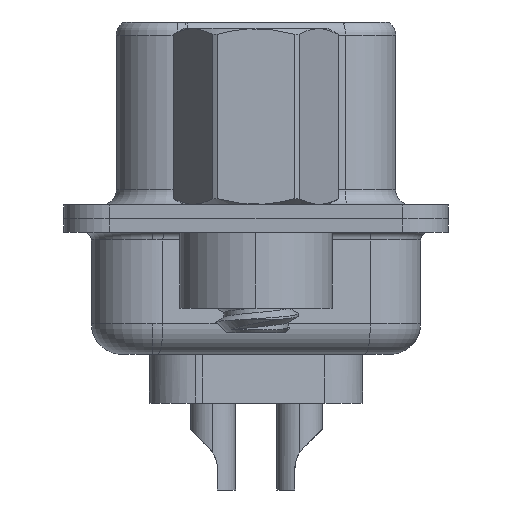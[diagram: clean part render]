
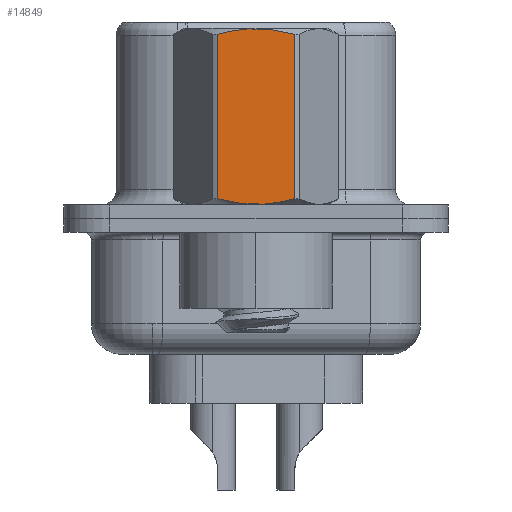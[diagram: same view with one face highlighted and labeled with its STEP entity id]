
A CAD part, left-side view. The second image highlights one B-rep face of the part: STEP entity #14849.
In plain terms, the highlighted planar face has unit normal (-1, 0, 0).
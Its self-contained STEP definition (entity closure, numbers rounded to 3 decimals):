
#554 = VECTOR ( 'NONE', #30911, 1000. ) ;
#1548 = ORIENTED_EDGE ( 'NONE', *, *, #30494, .T. ) ;
#2307 = DIRECTION ( 'NONE',  ( 0., -1., 0. ) ) ;
#3240 = VERTEX_POINT ( 'NONE', #31579 ) ;
#3548 = B_SPLINE_CURVE_WITH_KNOTS ( 'NONE', 3,
 ( #26288, #14529, #26446, #4551, #21928, #31749, #11772, #9682, #9529, #16793 ),
 .UNSPECIFIED., .F., .F.,
 ( 4, 2, 2, 2, 4 ),
 ( 0.001, 0.002, 0.002, 0.003, 0.004 ),
 .UNSPECIFIED. ) ;
#3938 = B_SPLINE_CURVE_WITH_KNOTS ( 'NONE', 3,
 ( #23975, #7053, #26225, #16888, #11562, #16259, #19156, #4168, #31684, #28947 ),
 .UNSPECIFIED., .F., .F.,
 ( 4, 2, 2, 2, 4 ),
 ( 0.003, 0.003, 0.004, 0.004, 0.005 ),
 .UNSPECIFIED. ) ;
#4168 = CARTESIAN_POINT ( 'NONE',  ( -2.381, -0.858, 0.55 ) ) ;
#4551 = CARTESIAN_POINT ( 'NONE',  ( -2.381, -0.432, 6.215 ) ) ;
#5986 = CARTESIAN_POINT ( 'NONE',  ( -2.381, 1.273, 3.792 ) ) ;
#6294 = ORIENTED_EDGE ( 'NONE', *, *, #14105, .T. ) ;
#7053 = CARTESIAN_POINT ( 'NONE',  ( -2.381, 1.065, 0.596 ) ) ;
#7662 = EDGE_LOOP ( 'NONE', ( #6294, #1548, #12717, #27139 ) ) ;
#9517 = PLANE ( 'NONE',  #10542 ) ;
#9529 = CARTESIAN_POINT ( 'NONE',  ( -2.381, 1.065, 6.104 ) ) ;
#9682 = CARTESIAN_POINT ( 'NONE',  ( -2.381, 0.853, 6.151 ) ) ;
#10542 = AXIS2_PLACEMENT_3D ( 'NONE', #26901, #29155, #2307 ) ;
#11562 = CARTESIAN_POINT ( 'NONE',  ( -2.381, 0.215, 0.468 ) ) ;
#11772 = CARTESIAN_POINT ( 'NONE',  ( -2.381, 0.428, 6.215 ) ) ;
#12717 = ORIENTED_EDGE ( 'NONE', *, *, #28779, .T. ) ;
#14105 = EDGE_CURVE ( 'NONE', #3240, #20142, #3938, .T. ) ;
#14252 = CARTESIAN_POINT ( 'NONE',  ( -2.381, -1.273, 6.048 ) ) ;
#14529 = CARTESIAN_POINT ( 'NONE',  ( -2.381, -1.066, 6.104 ) ) ;
#14849 = ADVANCED_FACE ( 'NONE', ( #19507 ), #9517, .T. ) ;
#15960 = LINE ( 'NONE', #5986, #554 ) ;
#15962 = CARTESIAN_POINT ( 'NONE',  ( -2.381, 1.273, 6.048 ) ) ;
#16259 = CARTESIAN_POINT ( 'NONE',  ( -2.381, -0.215, 0.468 ) ) ;
#16793 = CARTESIAN_POINT ( 'NONE',  ( -2.381, 1.273, 6.048 ) ) ;
#16868 = VERTEX_POINT ( 'NONE', #15962 ) ;
#16888 = CARTESIAN_POINT ( 'NONE',  ( -2.381, 0.428, 0.485 ) ) ;
#17293 = LINE ( 'NONE', #27558, #22139 ) ;
#18986 = CARTESIAN_POINT ( 'NONE',  ( -2.381, -1.273, 0.652 ) ) ;
#19156 = CARTESIAN_POINT ( 'NONE',  ( -2.381, -0.432, 0.485 ) ) ;
#19507 = FACE_OUTER_BOUND ( 'NONE', #7662, .T. ) ;
#20142 = VERTEX_POINT ( 'NONE', #18986 ) ;
#21928 = CARTESIAN_POINT ( 'NONE',  ( -2.381, -0.215, 6.232 ) ) ;
#22139 = VECTOR ( 'NONE', #27083, 1000. ) ;
#23975 = CARTESIAN_POINT ( 'NONE',  ( -2.381, 1.273, 0.652 ) ) ;
#25932 = VERTEX_POINT ( 'NONE', #14252 ) ;
#26225 = CARTESIAN_POINT ( 'NONE',  ( -2.381, 0.853, 0.549 ) ) ;
#26288 = CARTESIAN_POINT ( 'NONE',  ( -2.381, -1.273, 6.048 ) ) ;
#26446 = CARTESIAN_POINT ( 'NONE',  ( -2.381, -0.858, 6.15 ) ) ;
#26901 = CARTESIAN_POINT ( 'NONE',  ( -2.381, 1.375, -3.75 ) ) ;
#27083 = DIRECTION ( 'NONE',  ( 0., 0., 1. ) ) ;
#27139 = ORIENTED_EDGE ( 'NONE', *, *, #29092, .T. ) ;
#27558 = CARTESIAN_POINT ( 'NONE',  ( -2.381, -1.273, 3.792 ) ) ;
#28779 = EDGE_CURVE ( 'NONE', #25932, #16868, #3548, .T. ) ;
#28947 = CARTESIAN_POINT ( 'NONE',  ( -2.381, -1.273, 0.652 ) ) ;
#29092 = EDGE_CURVE ( 'NONE', #16868, #3240, #15960, .T. ) ;
#29155 = DIRECTION ( 'NONE',  ( -1., 0., 0. ) ) ;
#30494 = EDGE_CURVE ( 'NONE', #20142, #25932, #17293, .T. ) ;
#30911 = DIRECTION ( 'NONE',  ( 0., 0., -1. ) ) ;
#31579 = CARTESIAN_POINT ( 'NONE',  ( -2.381, 1.273, 0.652 ) ) ;
#31684 = CARTESIAN_POINT ( 'NONE',  ( -2.381, -1.066, 0.596 ) ) ;
#31749 = CARTESIAN_POINT ( 'NONE',  ( -2.381, 0.215, 6.232 ) ) ;
